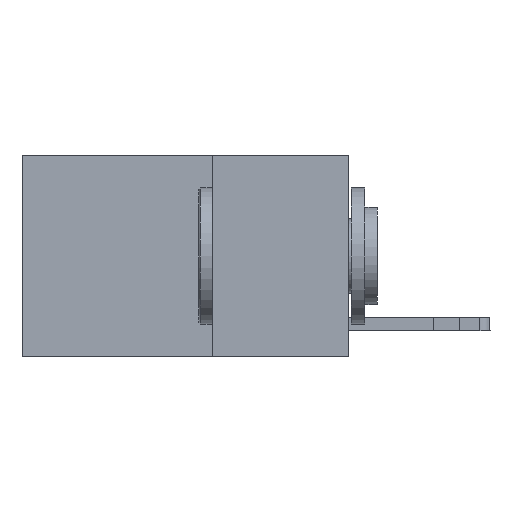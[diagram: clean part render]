
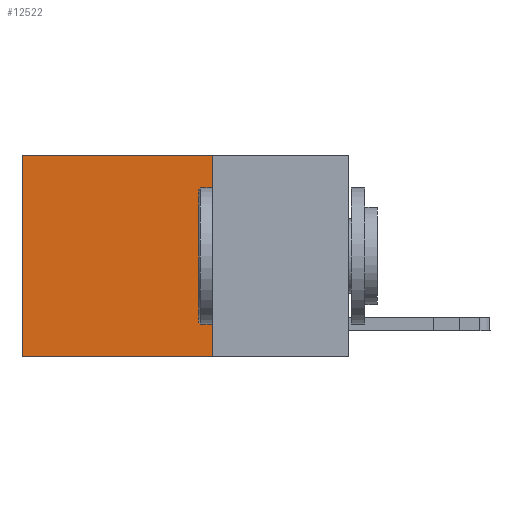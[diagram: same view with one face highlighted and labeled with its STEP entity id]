
A CAD part, left-side view. The second image highlights one B-rep face of the part: STEP entity #12522.
In plain terms, the highlighted planar face has unit normal (-1, 0, 0).
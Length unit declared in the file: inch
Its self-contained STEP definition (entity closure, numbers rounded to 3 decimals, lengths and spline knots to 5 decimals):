
#617 = VECTOR ( 'NONE', #15867, 39.37008 ) ;
#1246 = EDGE_CURVE ( 'NONE', #8215, #21602, #19962, .T. ) ;
#1819 = VECTOR ( 'NONE', #16718, 39.37008 ) ;
#2146 = EDGE_LOOP ( 'NONE', ( #7135, #22578, #15222, #23329 ) ) ;
#3449 = DIRECTION ( 'NONE',  ( 0., 0., -1. ) ) ;
#4802 = DIRECTION ( 'NONE',  ( 0., 0., -1. ) ) ;
#5355 = PLANE ( 'NONE',  #8249 ) ;
#6604 = DIRECTION ( 'NONE',  ( 0., 1., 0. ) ) ;
#7135 = ORIENTED_EDGE ( 'NONE', *, *, #24274, .T. ) ;
#7417 = CARTESIAN_POINT ( 'NONE',  ( 0.2625, 0.25, 0. ) ) ;
#7628 = CARTESIAN_POINT ( 'NONE',  ( 0.2625, 0.25, 0. ) ) ;
#7681 = DIRECTION ( 'NONE',  ( 1., 0., 0. ) ) ;
#8215 = VERTEX_POINT ( 'NONE', #12662 ) ;
#8249 = AXIS2_PLACEMENT_3D ( 'NONE', #7417, #7681, #3449 ) ;
#9702 = CARTESIAN_POINT ( 'NONE',  ( 0.2625, 0.6, 0. ) ) ;
#9897 = CARTESIAN_POINT ( 'NONE',  ( 0.2625, 0.6, -0.37 ) ) ;
#10594 = VERTEX_POINT ( 'NONE', #9897 ) ;
#10964 = LINE ( 'NONE', #25497, #1819 ) ;
#11559 = FACE_OUTER_BOUND ( 'NONE', #2146, .T. ) ;
#12263 = VECTOR ( 'NONE', #4802, 39.37008 ) ;
#12522 = ADVANCED_FACE ( 'NONE', ( #11559 ), #5355, .F. ) ;
#12662 = CARTESIAN_POINT ( 'NONE',  ( 0.2625, 0.25, 0. ) ) ;
#13315 = CARTESIAN_POINT ( 'NONE',  ( 0.2625, 0.6, 0. ) ) ;
#13395 = CARTESIAN_POINT ( 'NONE',  ( 0.2625, 0.25, -0.37 ) ) ;
#15222 = ORIENTED_EDGE ( 'NONE', *, *, #1246, .F. ) ;
#15867 = DIRECTION ( 'NONE',  ( 0., 0., -1. ) ) ;
#16718 = DIRECTION ( 'NONE',  ( 0., 1., 0. ) ) ;
#17012 = LINE ( 'NONE', #25391, #23262 ) ;
#18918 = VERTEX_POINT ( 'NONE', #9702 ) ;
#19962 = LINE ( 'NONE', #7628, #617 ) ;
#21393 = LINE ( 'NONE', #13315, #12263 ) ;
#21602 = VERTEX_POINT ( 'NONE', #13395 ) ;
#22578 = ORIENTED_EDGE ( 'NONE', *, *, #26071, .F. ) ;
#23262 = VECTOR ( 'NONE', #6604, 39.37008 ) ;
#23329 = ORIENTED_EDGE ( 'NONE', *, *, #25746, .T. ) ;
#24274 = EDGE_CURVE ( 'NONE', #18918, #10594, #21393, .T. ) ;
#25391 = CARTESIAN_POINT ( 'NONE',  ( 0.2625, 0.25, 0. ) ) ;
#25497 = CARTESIAN_POINT ( 'NONE',  ( 0.2625, 0.25, -0.37 ) ) ;
#25746 = EDGE_CURVE ( 'NONE', #8215, #18918, #17012, .T. ) ;
#26071 = EDGE_CURVE ( 'NONE', #21602, #10594, #10964, .T. ) ;
